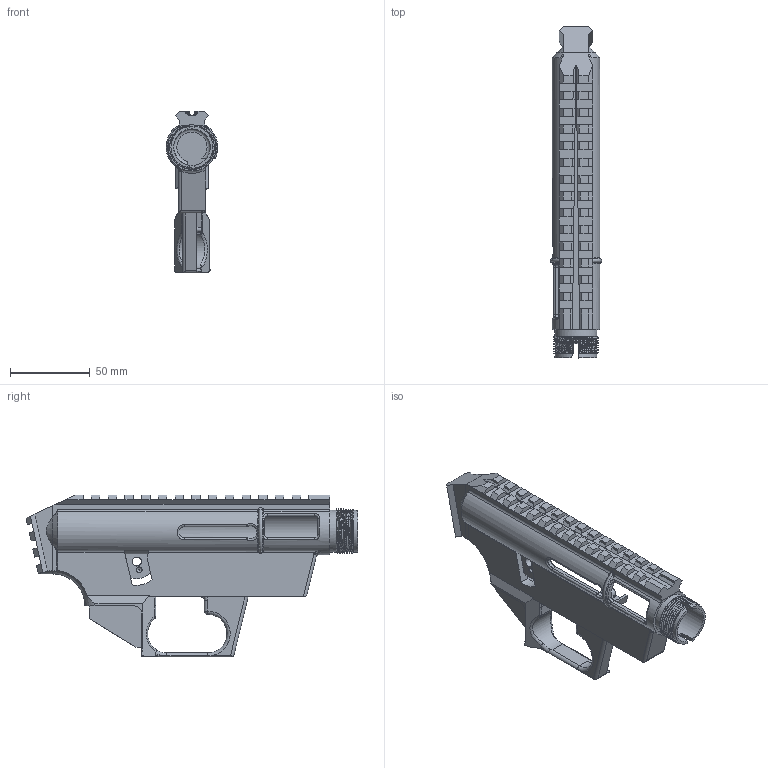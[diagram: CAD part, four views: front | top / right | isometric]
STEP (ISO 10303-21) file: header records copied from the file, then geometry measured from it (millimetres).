
FILE_DESCRIPTION(/* description */ (''),/* implementation_level */ '2;1');
FILE_NAME(/* name */ 'AR-7 Camper III v15.step',/* time_stamp */ '2021-01-02T23:57:03-05:00',/* author */ (''),/* organization */ (''),/* preprocessor_version */ 'ST-DEVELOPER v18.1',/* originating_system */ 'Autodesk Translation Framework v9.7.1.1290',/* authorisation */ '');
FILE_SCHEMA (('AUTOMOTIVE_DESIGN { 1 0 10303 214 3 1 1 }'));
Length unit declared in the file: millimetre
Products named in the file (2): AR-7 Camper III; Pistol Grip Assembly
Assembly tree (1 placements, depth 2):
  AR-7 Camper III
    Pistol Grip Assembly
Bounding box: 32.28 x 207.67 x 101.34 mm (x, y, z)
Volume: 134486.7 mm3; surface area: 55144 mm2
Topology: 2 solids, 2 shells, 588 faces, 1637 edges, 1051 vertices
Faces by surface type: plane 363, cylinder 127, bspline 63, torus 20, cone 11, sphere 4
Full cylindrical faces by diameter (mm): 3.45 x1, 3.75 x2, 3.95 x1, 4.3 x1, 5.65 x1, 5.9 x1, 7.75 x1, 22.9 x1, 26.132 x2, 26.3 x1, 27.85 x3
Entity records: 22712 total; most frequent: CARTESIAN_POINT 7999, ORIENTED_EDGE 3270, DIRECTION 2775, EDGE_CURVE 1635, LINE 1109, VECTOR 1109, VERTEX_POINT 1051, AXIS2_PLACEMENT_3D 833
